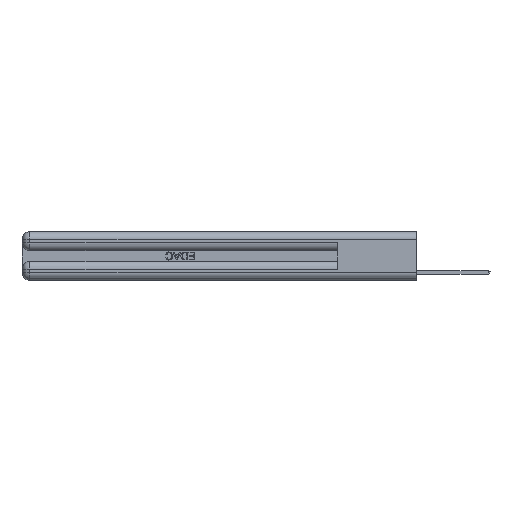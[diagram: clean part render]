
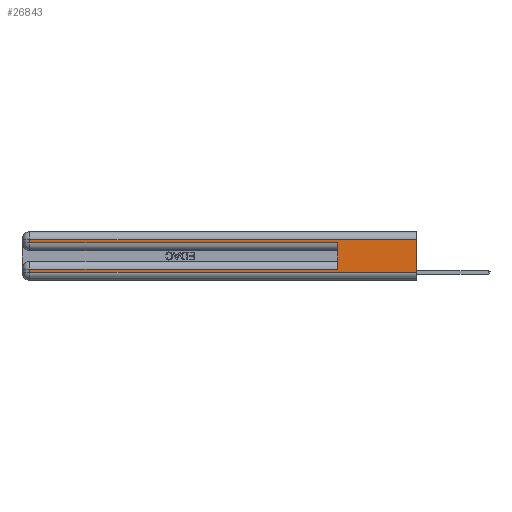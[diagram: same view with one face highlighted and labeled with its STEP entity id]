
A CAD part, left-side view. The second image highlights one B-rep face of the part: STEP entity #26843.
In plain terms, the highlighted planar face has unit normal (-1, 0, 0).
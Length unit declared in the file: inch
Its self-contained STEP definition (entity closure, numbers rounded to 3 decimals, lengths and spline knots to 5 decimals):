
#217 = CARTESIAN_POINT ( 'NONE',  ( 0., 0., 0.085 ) ) ;
#460 = DIRECTION ( 'NONE',  ( 0., 1., 0. ) ) ;
#1233 = VECTOR ( 'NONE', #3707, 39.37008 ) ;
#1628 = DIRECTION ( 'NONE',  ( 0., 0., -1. ) ) ;
#1684 = DIRECTION ( 'NONE',  ( 0., 0., -1. ) ) ;
#2040 = LINE ( 'NONE', #27994, #1233 ) ;
#2360 = LINE ( 'NONE', #25274, #8275 ) ;
#3092 = VERTEX_POINT ( 'NONE', #31720 ) ;
#3152 = VECTOR ( 'NONE', #5992, 39.37008 ) ;
#3707 = DIRECTION ( 'NONE',  ( 0., -1., 0. ) ) ;
#4288 = ORIENTED_EDGE ( 'NONE', *, *, #5752, .F. ) ;
#4807 = ORIENTED_EDGE ( 'NONE', *, *, #29075, .F. ) ;
#5324 = VERTEX_POINT ( 'NONE', #8361 ) ;
#5752 = EDGE_CURVE ( 'NONE', #5324, #3092, #29590, .T. ) ;
#5992 = DIRECTION ( 'NONE',  ( 0., 0., -1. ) ) ;
#6651 = VERTEX_POINT ( 'NONE', #20351 ) ;
#6661 = DIRECTION ( 'NONE',  ( 0., 0., -1. ) ) ;
#6754 = ORIENTED_EDGE ( 'NONE', *, *, #8224, .T. ) ;
#7339 = VECTOR ( 'NONE', #33957, 39.37008 ) ;
#7658 = VECTOR ( 'NONE', #7949, 39.37008 ) ;
#7747 = VERTEX_POINT ( 'NONE', #28130 ) ;
#7833 = ORIENTED_EDGE ( 'NONE', *, *, #31709, .T. ) ;
#7949 = DIRECTION ( 'NONE',  ( 0., -1., 0. ) ) ;
#8224 = EDGE_CURVE ( 'NONE', #6651, #28553, #24952, .T. ) ;
#8275 = VECTOR ( 'NONE', #6661, 39.37008 ) ;
#8361 = CARTESIAN_POINT ( 'NONE',  ( 0., 0.6, 0.085 ) ) ;
#8405 = ORIENTED_EDGE ( 'NONE', *, *, #30207, .T. ) ;
#9049 = VERTEX_POINT ( 'NONE', #31923 ) ;
#9053 = AXIS2_PLACEMENT_3D ( 'NONE', #17723, #20782, #1684 ) ;
#11426 = LINE ( 'NONE', #26826, #7658 ) ;
#12885 = CARTESIAN_POINT ( 'NONE',  ( 0., 0., 0.31 ) ) ;
#15059 = CARTESIAN_POINT ( 'NONE',  ( 0., 2.94, 0.31 ) ) ;
#15651 = VECTOR ( 'NONE', #460, 39.37008 ) ;
#16349 = CARTESIAN_POINT ( 'NONE',  ( 0., 2.94, 0.085 ) ) ;
#16741 = CARTESIAN_POINT ( 'NONE',  ( 0., 2.94, 0.37 ) ) ;
#17057 = ORIENTED_EDGE ( 'NONE', *, *, #19705, .T. ) ;
#17409 = LINE ( 'NONE', #23892, #3152 ) ;
#17635 = EDGE_CURVE ( 'NONE', #5324, #23292, #26176, .T. ) ;
#17723 = CARTESIAN_POINT ( 'NONE',  ( 0., 0., 0.37 ) ) ;
#18043 = CARTESIAN_POINT ( 'NONE',  ( 0., 0.6, 0.145 ) ) ;
#18961 = EDGE_LOOP ( 'NONE', ( #4807, #6754, #8405, #7833, #4288, #29936, #27158, #17057 ) ) ;
#19705 = EDGE_CURVE ( 'NONE', #28680, #7747, #2040, .T. ) ;
#20351 = CARTESIAN_POINT ( 'NONE',  ( 0., 0., 0.31 ) ) ;
#20570 = FACE_OUTER_BOUND ( 'NONE', #18961, .T. ) ;
#20782 = DIRECTION ( 'NONE',  ( 1., 0., 0. ) ) ;
#23292 = VERTEX_POINT ( 'NONE', #16349 ) ;
#23892 = CARTESIAN_POINT ( 'NONE',  ( 0., 2.94, 0.37 ) ) ;
#24003 = CARTESIAN_POINT ( 'NONE',  ( 0., 2.94, 0.06 ) ) ;
#24563 = VECTOR ( 'NONE', #25838, 39.37008 ) ;
#24952 = LINE ( 'NONE', #12885, #7339 ) ;
#25274 = CARTESIAN_POINT ( 'NONE',  ( 0., 0., 0.37 ) ) ;
#25838 = DIRECTION ( 'NONE',  ( 0., 0., 1. ) ) ;
#26176 = LINE ( 'NONE', #217, #15651 ) ;
#26826 = CARTESIAN_POINT ( 'NONE',  ( 0., 0., 0.285 ) ) ;
#26843 = ADVANCED_FACE ( 'NONE', ( #20570 ), #33908, .F. ) ;
#27158 = ORIENTED_EDGE ( 'NONE', *, *, #30091, .T. ) ;
#27994 = CARTESIAN_POINT ( 'NONE',  ( 0., 0., 0.06 ) ) ;
#28130 = CARTESIAN_POINT ( 'NONE',  ( 0., 0., 0.06 ) ) ;
#28553 = VERTEX_POINT ( 'NONE', #15059 ) ;
#28680 = VERTEX_POINT ( 'NONE', #24003 ) ;
#29075 = EDGE_CURVE ( 'NONE', #6651, #7747, #2360, .T. ) ;
#29570 = LINE ( 'NONE', #16741, #30413 ) ;
#29590 = LINE ( 'NONE', #18043, #24563 ) ;
#29936 = ORIENTED_EDGE ( 'NONE', *, *, #17635, .T. ) ;
#30091 = EDGE_CURVE ( 'NONE', #23292, #28680, #17409, .T. ) ;
#30207 = EDGE_CURVE ( 'NONE', #28553, #9049, #29570, .T. ) ;
#30413 = VECTOR ( 'NONE', #1628, 39.37008 ) ;
#31709 = EDGE_CURVE ( 'NONE', #9049, #3092, #11426, .T. ) ;
#31720 = CARTESIAN_POINT ( 'NONE',  ( 0., 0.6, 0.285 ) ) ;
#31923 = CARTESIAN_POINT ( 'NONE',  ( 0., 2.94, 0.285 ) ) ;
#33908 = PLANE ( 'NONE',  #9053 ) ;
#33957 = DIRECTION ( 'NONE',  ( 0., 1., 0. ) ) ;
